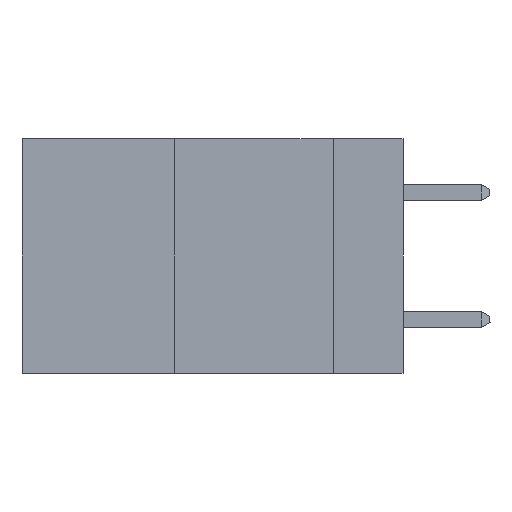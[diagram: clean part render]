
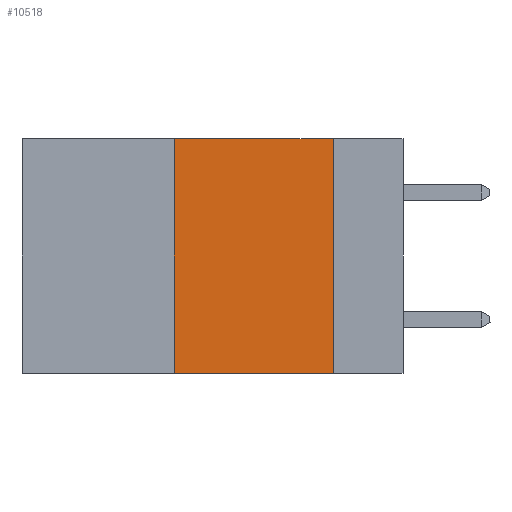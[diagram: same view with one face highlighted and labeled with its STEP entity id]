
A CAD part, left-side view. The second image highlights one B-rep face of the part: STEP entity #10518.
In plain terms, the highlighted planar face has unit normal (-1, 0, 0).
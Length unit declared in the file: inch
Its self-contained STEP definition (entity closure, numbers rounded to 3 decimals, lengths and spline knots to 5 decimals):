
#620 = EDGE_CURVE ( 'NONE', #15438, #14538, #7876, .T. ) ;
#636 = VECTOR ( 'NONE', #9221, 39.37008 ) ;
#912 = CARTESIAN_POINT ( 'NONE',  ( 0., 0.11, -0.37 ) ) ;
#1935 = PLANE ( 'NONE',  #16048 ) ;
#2116 = CARTESIAN_POINT ( 'NONE',  ( 0., 0.6, 0. ) ) ;
#2796 = VECTOR ( 'NONE', #9623, 39.37008 ) ;
#4722 = DIRECTION ( 'NONE',  ( 0., -1., 0. ) ) ;
#5252 = EDGE_CURVE ( 'NONE', #9694, #15727, #10221, .T. ) ;
#5490 = CARTESIAN_POINT ( 'NONE',  ( 0., 0.36, -0.37 ) ) ;
#5799 = ORIENTED_EDGE ( 'NONE', *, *, #13040, .T. ) ;
#5909 = ORIENTED_EDGE ( 'NONE', *, *, #5252, .F. ) ;
#6210 = DIRECTION ( 'NONE',  ( 0., 0., -1. ) ) ;
#6853 = CARTESIAN_POINT ( 'NONE',  ( 0., 0.36, 0. ) ) ;
#6856 = ORIENTED_EDGE ( 'NONE', *, *, #620, .F. ) ;
#7225 = LINE ( 'NONE', #8812, #15942 ) ;
#7876 = LINE ( 'NONE', #17531, #636 ) ;
#8812 = CARTESIAN_POINT ( 'NONE',  ( 0., 0.6, -0.37 ) ) ;
#9097 = CARTESIAN_POINT ( 'NONE',  ( 0., 0.36, 0. ) ) ;
#9221 = DIRECTION ( 'NONE',  ( 0., 0., -1. ) ) ;
#9623 = DIRECTION ( 'NONE',  ( 0., 0., 1. ) ) ;
#9694 = VERTEX_POINT ( 'NONE', #5490 ) ;
#10221 = LINE ( 'NONE', #6853, #2796 ) ;
#10518 = ADVANCED_FACE ( 'NONE', ( #14586 ), #1935, .F. ) ;
#10626 = EDGE_LOOP ( 'NONE', ( #6856, #14782, #5909, #5799 ) ) ;
#11615 = LINE ( 'NONE', #13856, #16607 ) ;
#12120 = EDGE_CURVE ( 'NONE', #15727, #15438, #11615, .T. ) ;
#12386 = DIRECTION ( 'NONE',  ( 0., -1., 0. ) ) ;
#13040 = EDGE_CURVE ( 'NONE', #9694, #14538, #7225, .T. ) ;
#13856 = CARTESIAN_POINT ( 'NONE',  ( 0., 0.6, 0. ) ) ;
#13926 = CARTESIAN_POINT ( 'NONE',  ( 0., 0.11, 0. ) ) ;
#14538 = VERTEX_POINT ( 'NONE', #912 ) ;
#14586 = FACE_OUTER_BOUND ( 'NONE', #10626, .T. ) ;
#14782 = ORIENTED_EDGE ( 'NONE', *, *, #12120, .F. ) ;
#15438 = VERTEX_POINT ( 'NONE', #13926 ) ;
#15727 = VERTEX_POINT ( 'NONE', #9097 ) ;
#15942 = VECTOR ( 'NONE', #4722, 39.37008 ) ;
#16048 = AXIS2_PLACEMENT_3D ( 'NONE', #2116, #17358, #6210 ) ;
#16607 = VECTOR ( 'NONE', #12386, 39.37008 ) ;
#17358 = DIRECTION ( 'NONE',  ( 1., 0., 0. ) ) ;
#17531 = CARTESIAN_POINT ( 'NONE',  ( 0., 0.11, 0. ) ) ;
